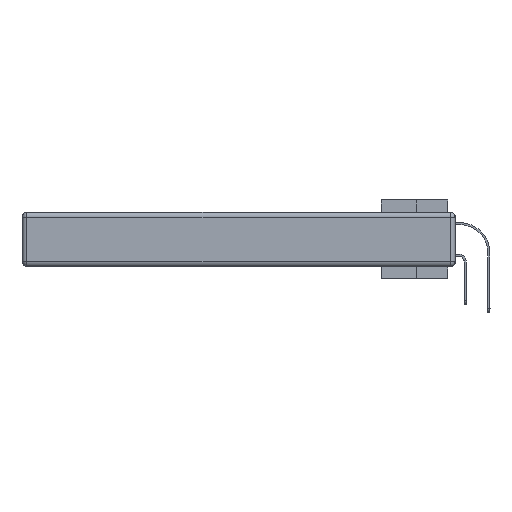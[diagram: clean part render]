
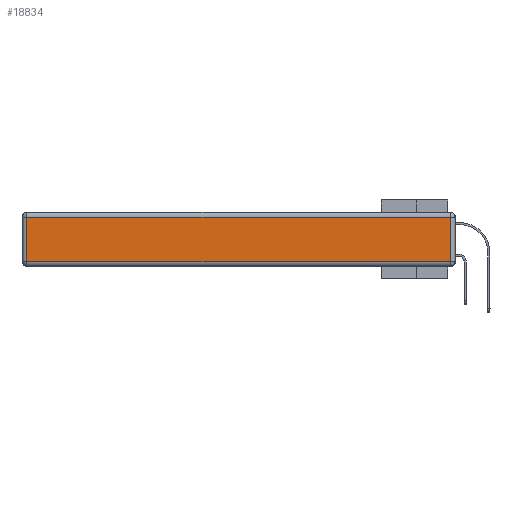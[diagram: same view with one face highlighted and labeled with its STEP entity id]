
A CAD part, left-side view. The second image highlights one B-rep face of the part: STEP entity #18834.
In plain terms, the highlighted planar face has unit normal (-1, 0, 0).
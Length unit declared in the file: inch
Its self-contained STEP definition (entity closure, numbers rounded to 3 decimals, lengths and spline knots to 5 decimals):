
#26 = FACE_OUTER_BOUND ( 'NONE', #15990, .T. ) ;
#2512 = CARTESIAN_POINT ( 'NONE',  ( 0., 2.75, -0.03 ) ) ;
#2751 = CARTESIAN_POINT ( 'NONE',  ( 0., 0., -0.343 ) ) ;
#5312 = EDGE_CURVE ( 'NONE', #18428, #17193, #26734, .T. ) ;
#6107 = DIRECTION ( 'NONE',  ( -1., 0., 0. ) ) ;
#6894 = VERTEX_POINT ( 'NONE', #6906 ) ;
#6906 = CARTESIAN_POINT ( 'NONE',  ( 0., 0.03, -0.313 ) ) ;
#9727 = DIRECTION ( 'NONE',  ( 0., -1., 0. ) ) ;
#10085 = VECTOR ( 'NONE', #9727, 39.37008 ) ;
#11117 = CARTESIAN_POINT ( 'NONE',  ( 0., 2.72, -0.313 ) ) ;
#11448 = EDGE_CURVE ( 'NONE', #38453, #18428, #24437, .T. ) ;
#15990 = EDGE_LOOP ( 'NONE', ( #26997, #32159, #22891, #29974 ) ) ;
#17193 = VERTEX_POINT ( 'NONE', #11117 ) ;
#18428 = VERTEX_POINT ( 'NONE', #25119 ) ;
#18834 = ADVANCED_FACE ( 'NONE', ( #26 ), #41073, .T. ) ;
#18973 = DIRECTION ( 'NONE',  ( 0., 0., 1. ) ) ;
#19444 = CARTESIAN_POINT ( 'NONE',  ( 0., 0., -0.313 ) ) ;
#20634 = VECTOR ( 'NONE', #38107, 39.37008 ) ;
#22805 = LINE ( 'NONE', #19444, #10085 ) ;
#22891 = ORIENTED_EDGE ( 'NONE', *, *, #11448, .T. ) ;
#23978 = CARTESIAN_POINT ( 'NONE',  ( 0., 2.72, -0.343 ) ) ;
#24437 = LINE ( 'NONE', #2512, #20634 ) ;
#24539 = CARTESIAN_POINT ( 'NONE',  ( 0., 0.03, -0.343 ) ) ;
#25119 = CARTESIAN_POINT ( 'NONE',  ( 0., 2.72, -0.03 ) ) ;
#25171 = DIRECTION ( 'NONE',  ( 0., 0., 1. ) ) ;
#25443 = EDGE_CURVE ( 'NONE', #17193, #6894, #22805, .T. ) ;
#26734 = LINE ( 'NONE', #23978, #31365 ) ;
#26997 = ORIENTED_EDGE ( 'NONE', *, *, #25443, .T. ) ;
#28869 = VECTOR ( 'NONE', #25171, 39.37008 ) ;
#29974 = ORIENTED_EDGE ( 'NONE', *, *, #5312, .T. ) ;
#31365 = VECTOR ( 'NONE', #40213, 39.37008 ) ;
#32159 = ORIENTED_EDGE ( 'NONE', *, *, #41090, .T. ) ;
#37828 = LINE ( 'NONE', #24539, #28869 ) ;
#38107 = DIRECTION ( 'NONE',  ( 0., 1., 0. ) ) ;
#38453 = VERTEX_POINT ( 'NONE', #41525 ) ;
#39023 = AXIS2_PLACEMENT_3D ( 'NONE', #2751, #6107, #18973 ) ;
#40213 = DIRECTION ( 'NONE',  ( 0., 0., -1. ) ) ;
#41073 = PLANE ( 'NONE',  #39023 ) ;
#41090 = EDGE_CURVE ( 'NONE', #6894, #38453, #37828, .T. ) ;
#41525 = CARTESIAN_POINT ( 'NONE',  ( 0., 0.03, -0.03 ) ) ;
